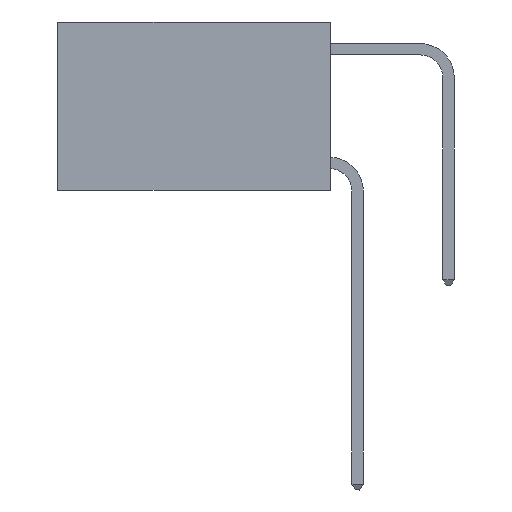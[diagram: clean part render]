
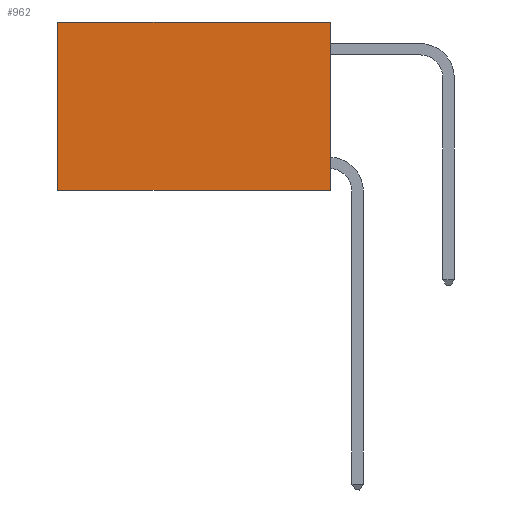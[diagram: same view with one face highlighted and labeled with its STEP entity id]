
A CAD part, left-side view. The second image highlights one B-rep face of the part: STEP entity #962.
In plain terms, the highlighted planar face has unit normal (-1, 0, 0).
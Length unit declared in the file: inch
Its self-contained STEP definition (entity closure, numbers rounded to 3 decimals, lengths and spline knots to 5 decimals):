
#558 = EDGE_CURVE ( 'NONE', #18600, #2339, #2083, .T. ) ;
#774 = CARTESIAN_POINT ( 'NONE',  ( 0.2625, 0.6, -0.37 ) ) ;
#889 = CARTESIAN_POINT ( 'NONE',  ( 0.2625, 0., -0.37 ) ) ;
#937 = DIRECTION ( 'NONE',  ( 0., 1., 0. ) ) ;
#962 = ADVANCED_FACE ( 'NONE', ( #22224 ), #5495, .F. ) ;
#1056 = EDGE_LOOP ( 'NONE', ( #13175, #14565, #13319, #2016 ) ) ;
#2016 = ORIENTED_EDGE ( 'NONE', *, *, #3877, .T. ) ;
#2055 = DIRECTION ( 'NONE',  ( 1., 0., 0. ) ) ;
#2083 = LINE ( 'NONE', #13143, #6783 ) ;
#2339 = VERTEX_POINT ( 'NONE', #774 ) ;
#2648 = LINE ( 'NONE', #17782, #9432 ) ;
#3877 = EDGE_CURVE ( 'NONE', #7348, #15090, #2648, .T. ) ;
#3881 = CARTESIAN_POINT ( 'NONE',  ( 0.2625, 0., 0. ) ) ;
#5495 = PLANE ( 'NONE',  #7218 ) ;
#6026 = CARTESIAN_POINT ( 'NONE',  ( 0.2625, 0.6, 0. ) ) ;
#6783 = VECTOR ( 'NONE', #15005, 39.37008 ) ;
#7218 = AXIS2_PLACEMENT_3D ( 'NONE', #3881, #2055, #9544 ) ;
#7348 = VERTEX_POINT ( 'NONE', #17041 ) ;
#9432 = VECTOR ( 'NONE', #937, 39.37008 ) ;
#9544 = DIRECTION ( 'NONE',  ( 0., 0., -1. ) ) ;
#9762 = EDGE_CURVE ( 'NONE', #15090, #2339, #10410, .T. ) ;
#10410 = LINE ( 'NONE', #6026, #23406 ) ;
#11985 = DIRECTION ( 'NONE',  ( 0., 0., -1. ) ) ;
#13143 = CARTESIAN_POINT ( 'NONE',  ( 0.2625, 0., -0.37 ) ) ;
#13175 = ORIENTED_EDGE ( 'NONE', *, *, #9762, .T. ) ;
#13319 = ORIENTED_EDGE ( 'NONE', *, *, #18203, .F. ) ;
#13727 = CARTESIAN_POINT ( 'NONE',  ( 0.2625, 0.6, 0. ) ) ;
#14109 = DIRECTION ( 'NONE',  ( 0., 0., -1. ) ) ;
#14565 = ORIENTED_EDGE ( 'NONE', *, *, #558, .F. ) ;
#14600 = VECTOR ( 'NONE', #11985, 39.37008 ) ;
#15005 = DIRECTION ( 'NONE',  ( 0., 1., 0. ) ) ;
#15090 = VERTEX_POINT ( 'NONE', #13727 ) ;
#17041 = CARTESIAN_POINT ( 'NONE',  ( 0.2625, 0., 0. ) ) ;
#17534 = CARTESIAN_POINT ( 'NONE',  ( 0.2625, 0., 0. ) ) ;
#17782 = CARTESIAN_POINT ( 'NONE',  ( 0.2625, 0., 0. ) ) ;
#18203 = EDGE_CURVE ( 'NONE', #7348, #18600, #22942, .T. ) ;
#18600 = VERTEX_POINT ( 'NONE', #889 ) ;
#22224 = FACE_OUTER_BOUND ( 'NONE', #1056, .T. ) ;
#22942 = LINE ( 'NONE', #17534, #14600 ) ;
#23406 = VECTOR ( 'NONE', #14109, 39.37008 ) ;
